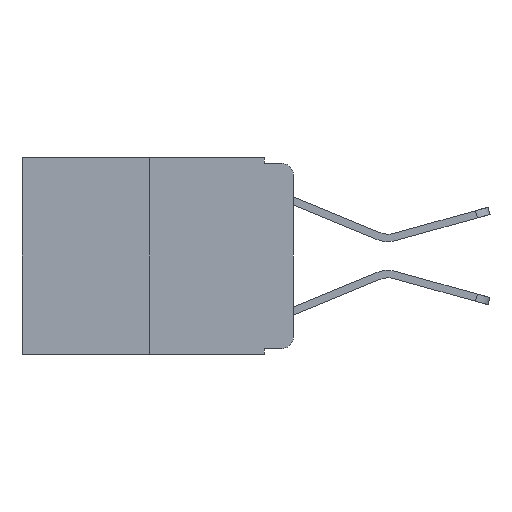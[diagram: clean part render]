
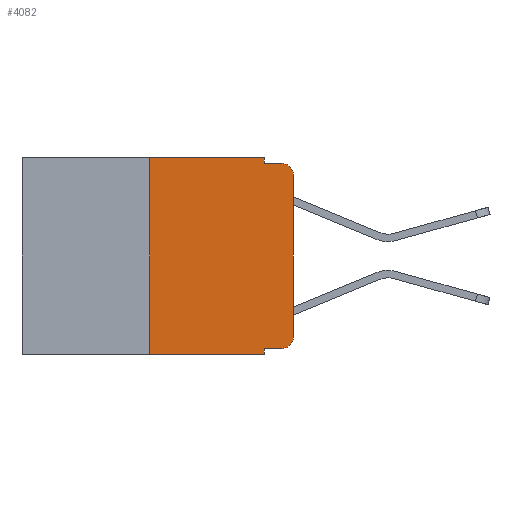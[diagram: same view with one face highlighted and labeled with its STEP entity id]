
A CAD part, left-side view. The second image highlights one B-rep face of the part: STEP entity #4082.
In plain terms, the highlighted planar face has unit normal (-1, 0, 0).
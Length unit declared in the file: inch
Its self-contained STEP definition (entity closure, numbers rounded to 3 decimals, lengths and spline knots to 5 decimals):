
#14 = ORIENTED_EDGE ( 'NONE', *, *, #7154, .F. ) ;
#115 = EDGE_CURVE ( 'NONE', #12166, #12176, #11862, .T. ) ;
#463 = ORIENTED_EDGE ( 'NONE', *, *, #17371, .T. ) ;
#511 = ORIENTED_EDGE ( 'NONE', *, *, #15195, .T. ) ;
#1083 = ORIENTED_EDGE ( 'NONE', *, *, #115, .F. ) ;
#1152 = DIRECTION ( 'NONE',  ( -1., 0., 0. ) ) ;
#1227 = VECTOR ( 'NONE', #12537, 39.37008 ) ;
#1589 = ORIENTED_EDGE ( 'NONE', *, *, #12358, .T. ) ;
#1648 = PLANE ( 'NONE',  #10562 ) ;
#1824 = VERTEX_POINT ( 'NONE', #4115 ) ;
#1838 = CARTESIAN_POINT ( 'NONE',  ( 0., 0.473, 0. ) ) ;
#2264 = EDGE_CURVE ( 'NONE', #8192, #14577, #15791, .T. ) ;
#2282 = CARTESIAN_POINT ( 'NONE',  ( 0., 0.25, -0.343 ) ) ;
#2345 = CARTESIAN_POINT ( 'NONE',  ( 0., 0.02, -0.03 ) ) ;
#2566 = ORIENTED_EDGE ( 'NONE', *, *, #15469, .F. ) ;
#2633 = DIRECTION ( 'NONE',  ( 0., -1., 0. ) ) ;
#3019 = ORIENTED_EDGE ( 'NONE', *, *, #7739, .T. ) ;
#3101 = DIRECTION ( 'NONE',  ( 0., 0., -1. ) ) ;
#3239 = LINE ( 'NONE', #11272, #10694 ) ;
#3441 = CARTESIAN_POINT ( 'NONE',  ( 0., 0.051, 0. ) ) ;
#3634 = CARTESIAN_POINT ( 'NONE',  ( 0., 0.051, -0.333 ) ) ;
#3869 = DIRECTION ( 'NONE',  ( 0., -1., 0. ) ) ;
#3910 = DIRECTION ( 'NONE',  ( 0., 0., -1. ) ) ;
#4082 = ADVANCED_FACE ( 'NONE', ( #12150 ), #1648, .F. ) ;
#4115 = CARTESIAN_POINT ( 'NONE',  ( 0., 0.02, -0.333 ) ) ;
#4268 = ORIENTED_EDGE ( 'NONE', *, *, #15324, .T. ) ;
#4353 = DIRECTION ( 'NONE',  ( 0., 0., -1. ) ) ;
#5174 = VERTEX_POINT ( 'NONE', #3634 ) ;
#5277 = ORIENTED_EDGE ( 'NONE', *, *, #2264, .F. ) ;
#5392 = DIRECTION ( 'NONE',  ( 0., -1., 0. ) ) ;
#5482 = LINE ( 'NONE', #16116, #16162 ) ;
#6181 = LINE ( 'NONE', #16979, #9647 ) ;
#6886 = AXIS2_PLACEMENT_3D ( 'NONE', #2345, #12766, #3910 ) ;
#7028 = CARTESIAN_POINT ( 'NONE',  ( 0., 0.25, 0. ) ) ;
#7154 = EDGE_CURVE ( 'NONE', #12176, #8192, #3239, .T. ) ;
#7339 = VECTOR ( 'NONE', #2633, 39.37008 ) ;
#7739 = EDGE_CURVE ( 'NONE', #13528, #14162, #9744, .T. ) ;
#7970 = VECTOR ( 'NONE', #17017, 39.37008 ) ;
#8118 = VERTEX_POINT ( 'NONE', #16474 ) ;
#8192 = VERTEX_POINT ( 'NONE', #3441 ) ;
#8207 = AXIS2_PLACEMENT_3D ( 'NONE', #10198, #1152, #11702 ) ;
#8360 = CARTESIAN_POINT ( 'NONE',  ( 0., 0.25, 0. ) ) ;
#9105 = CIRCLE ( 'NONE', #6886, 0.02 ) ;
#9496 = EDGE_LOOP ( 'NONE', ( #3019, #463, #2566, #5277, #14, #1083, #4268, #15825, #511, #1589 ) ) ;
#9647 = VECTOR ( 'NONE', #5392, 39.37008 ) ;
#9744 = LINE ( 'NONE', #11060, #1227 ) ;
#10078 = CARTESIAN_POINT ( 'NONE',  ( 0., 0.473, -0.343 ) ) ;
#10198 = CARTESIAN_POINT ( 'NONE',  ( 0., 0.02, -0.313 ) ) ;
#10562 = AXIS2_PLACEMENT_3D ( 'NONE', #1838, #15449, #3101 ) ;
#10694 = VECTOR ( 'NONE', #3869, 39.37008 ) ;
#11060 = CARTESIAN_POINT ( 'NONE',  ( 0., 0., 0. ) ) ;
#11272 = CARTESIAN_POINT ( 'NONE',  ( 0., 0.473, 0. ) ) ;
#11288 = EDGE_CURVE ( 'NONE', #5174, #8118, #15295, .T. ) ;
#11411 = CARTESIAN_POINT ( 'NONE',  ( 0., 0.051, -0.01 ) ) ;
#11523 = VECTOR ( 'NONE', #14755, 39.37008 ) ;
#11546 = CARTESIAN_POINT ( 'NONE',  ( 0., 0.051, 0. ) ) ;
#11702 = DIRECTION ( 'NONE',  ( 0., 0., -1. ) ) ;
#11862 = LINE ( 'NONE', #7028, #7970 ) ;
#12009 = VECTOR ( 'NONE', #4353, 39.37008 ) ;
#12150 = FACE_OUTER_BOUND ( 'NONE', #9496, .T. ) ;
#12166 = VERTEX_POINT ( 'NONE', #2282 ) ;
#12176 = VERTEX_POINT ( 'NONE', #8360 ) ;
#12358 = EDGE_CURVE ( 'NONE', #1824, #13528, #15483, .T. ) ;
#12537 = DIRECTION ( 'NONE',  ( 0., 0., 1. ) ) ;
#12766 = DIRECTION ( 'NONE',  ( -1., 0., 0. ) ) ;
#12884 = CARTESIAN_POINT ( 'NONE',  ( 0., 0., -0.03 ) ) ;
#13358 = CARTESIAN_POINT ( 'NONE',  ( 0., 0.051, 0. ) ) ;
#13528 = VERTEX_POINT ( 'NONE', #18459 ) ;
#14162 = VERTEX_POINT ( 'NONE', #12884 ) ;
#14577 = VERTEX_POINT ( 'NONE', #11411 ) ;
#14755 = DIRECTION ( 'NONE',  ( 0., 0., -1. ) ) ;
#15042 = LINE ( 'NONE', #10078, #7339 ) ;
#15121 = CARTESIAN_POINT ( 'NONE',  ( 0., 0.02, -0.01 ) ) ;
#15195 = EDGE_CURVE ( 'NONE', #5174, #1824, #6181, .T. ) ;
#15295 = LINE ( 'NONE', #13358, #11523 ) ;
#15324 = EDGE_CURVE ( 'NONE', #12166, #8118, #15042, .T. ) ;
#15449 = DIRECTION ( 'NONE',  ( 1., 0., 0. ) ) ;
#15469 = EDGE_CURVE ( 'NONE', #14577, #18990, #5482, .T. ) ;
#15483 = CIRCLE ( 'NONE', #8207, 0.02 ) ;
#15791 = LINE ( 'NONE', #11546, #12009 ) ;
#15825 = ORIENTED_EDGE ( 'NONE', *, *, #11288, .F. ) ;
#16116 = CARTESIAN_POINT ( 'NONE',  ( 0., 0.051, -0.01 ) ) ;
#16162 = VECTOR ( 'NONE', #18932, 39.37008 ) ;
#16474 = CARTESIAN_POINT ( 'NONE',  ( 0., 0.051, -0.343 ) ) ;
#16979 = CARTESIAN_POINT ( 'NONE',  ( 0., 0.051, -0.333 ) ) ;
#17017 = DIRECTION ( 'NONE',  ( 0., 0., 1. ) ) ;
#17371 = EDGE_CURVE ( 'NONE', #14162, #18990, #9105, .T. ) ;
#18459 = CARTESIAN_POINT ( 'NONE',  ( 0., 0., -0.313 ) ) ;
#18932 = DIRECTION ( 'NONE',  ( 0., -1., 0. ) ) ;
#18990 = VERTEX_POINT ( 'NONE', #15121 ) ;
